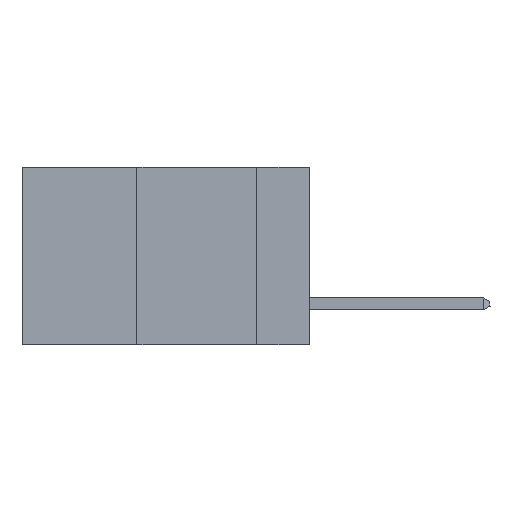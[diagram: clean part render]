
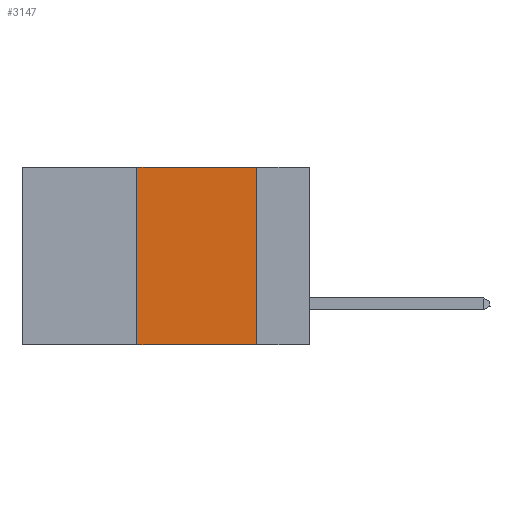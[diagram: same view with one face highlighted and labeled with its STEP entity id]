
A CAD part, left-side view. The second image highlights one B-rep face of the part: STEP entity #3147.
In plain terms, the highlighted planar face has unit normal (-1, 0, 0).
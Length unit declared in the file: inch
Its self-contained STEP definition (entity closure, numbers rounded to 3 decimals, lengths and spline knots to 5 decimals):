
#714 = DIRECTION ( 'NONE',  ( 0., -1., 0. ) ) ;
#1511 = VERTEX_POINT ( 'NONE', #15725 ) ;
#1553 = ORIENTED_EDGE ( 'NONE', *, *, #21417, .F. ) ;
#1607 = AXIS2_PLACEMENT_3D ( 'NONE', #24682, #22935, #9414 ) ;
#1909 = CARTESIAN_POINT ( 'NONE',  ( 0., 0.36, 0. ) ) ;
#2023 = ORIENTED_EDGE ( 'NONE', *, *, #3637, .F. ) ;
#3147 = ADVANCED_FACE ( 'NONE', ( #20629 ), #20968, .F. ) ;
#3637 = EDGE_CURVE ( 'NONE', #1511, #15835, #24482, .T. ) ;
#3881 = VECTOR ( 'NONE', #14958, 39.37008 ) ;
#5051 = VERTEX_POINT ( 'NONE', #1909 ) ;
#5860 = ORIENTED_EDGE ( 'NONE', *, *, #16682, .T. ) ;
#6083 = CARTESIAN_POINT ( 'NONE',  ( 0., 0.36, -0.37 ) ) ;
#9370 = CARTESIAN_POINT ( 'NONE',  ( 0., 0.11, 0. ) ) ;
#9414 = DIRECTION ( 'NONE',  ( 0., 0., -1. ) ) ;
#9793 = ORIENTED_EDGE ( 'NONE', *, *, #19268, .F. ) ;
#10154 = LINE ( 'NONE', #11017, #3881 ) ;
#11017 = CARTESIAN_POINT ( 'NONE',  ( 0., 0.36, 0. ) ) ;
#11490 = VECTOR ( 'NONE', #13450, 39.37008 ) ;
#13113 = VECTOR ( 'NONE', #17013, 39.37008 ) ;
#13135 = CARTESIAN_POINT ( 'NONE',  ( 0., 0.6, 0. ) ) ;
#13450 = DIRECTION ( 'NONE',  ( 0., 0., -1. ) ) ;
#13529 = CARTESIAN_POINT ( 'NONE',  ( 0., 0.11, -0.37 ) ) ;
#14958 = DIRECTION ( 'NONE',  ( 0., 0., 1. ) ) ;
#15725 = CARTESIAN_POINT ( 'NONE',  ( 0., 0.11, 0. ) ) ;
#15835 = VERTEX_POINT ( 'NONE', #13529 ) ;
#16682 = EDGE_CURVE ( 'NONE', #23524, #15835, #24936, .T. ) ;
#17013 = DIRECTION ( 'NONE',  ( 0., -1., 0. ) ) ;
#19125 = EDGE_LOOP ( 'NONE', ( #2023, #1553, #9793, #5860 ) ) ;
#19268 = EDGE_CURVE ( 'NONE', #23524, #5051, #10154, .T. ) ;
#19789 = VECTOR ( 'NONE', #714, 39.37008 ) ;
#20629 = FACE_OUTER_BOUND ( 'NONE', #19125, .T. ) ;
#20968 = PLANE ( 'NONE',  #1607 ) ;
#21417 = EDGE_CURVE ( 'NONE', #5051, #1511, #23119, .T. ) ;
#22051 = CARTESIAN_POINT ( 'NONE',  ( 0., 0.6, -0.37 ) ) ;
#22935 = DIRECTION ( 'NONE',  ( 1., 0., 0. ) ) ;
#23119 = LINE ( 'NONE', #13135, #13113 ) ;
#23524 = VERTEX_POINT ( 'NONE', #6083 ) ;
#24482 = LINE ( 'NONE', #9370, #11490 ) ;
#24682 = CARTESIAN_POINT ( 'NONE',  ( 0., 0.6, 0. ) ) ;
#24936 = LINE ( 'NONE', #22051, #19789 ) ;
